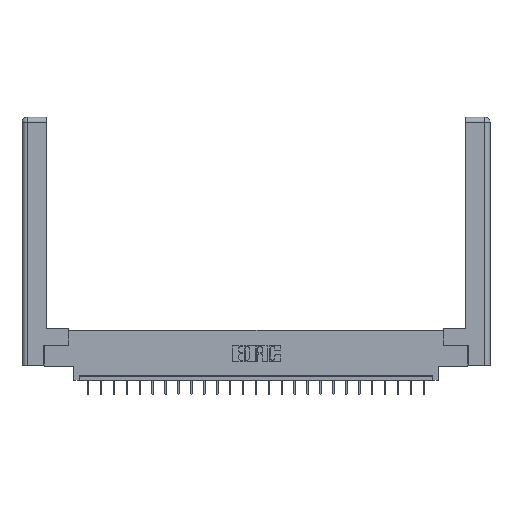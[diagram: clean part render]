
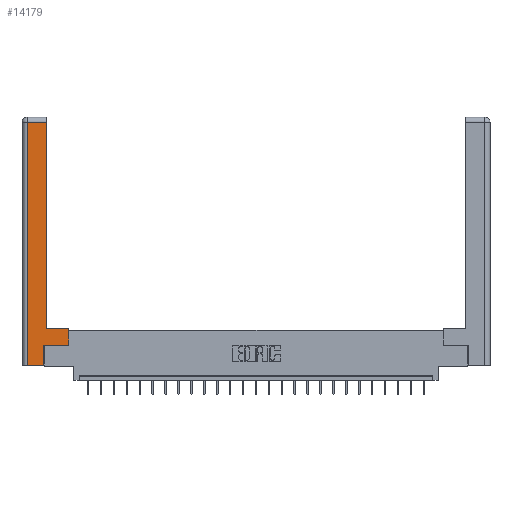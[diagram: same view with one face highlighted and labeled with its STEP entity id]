
A CAD part, top view. The second image highlights one B-rep face of the part: STEP entity #14179.
In plain terms, the highlighted planar face has unit normal (0, 0, 1).
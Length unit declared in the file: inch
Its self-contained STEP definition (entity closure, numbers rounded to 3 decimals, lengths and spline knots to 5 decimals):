
#237 = ORIENTED_EDGE ( 'NONE', *, *, #5616, .T. ) ;
#306 = CARTESIAN_POINT ( 'NONE',  ( 0.265, 0.245, 0. ) ) ;
#751 = VECTOR ( 'NONE', #7410, 39.37008 ) ;
#1029 = VECTOR ( 'NONE', #24122, 39.37008 ) ;
#1068 = VERTEX_POINT ( 'NONE', #18062 ) ;
#2059 = ORIENTED_EDGE ( 'NONE', *, *, #8962, .T. ) ;
#2095 = DIRECTION ( 'NONE',  ( -1., 0., 0. ) ) ;
#2140 = LINE ( 'NONE', #4128, #20501 ) ;
#3215 = FACE_OUTER_BOUND ( 'NONE', #4001, .T. ) ;
#3559 = DIRECTION ( 'NONE',  ( 1., 0., 0. ) ) ;
#3942 = LINE ( 'NONE', #7046, #16914 ) ;
#4001 = EDGE_LOOP ( 'NONE', ( #12333, #2059, #17284, #21267, #6269, #237, #24018, #21779 ) ) ;
#4022 = VECTOR ( 'NONE', #21543, 39.37008 ) ;
#4128 = CARTESIAN_POINT ( 'NONE',  ( 0.0615, 2.94, 0. ) ) ;
#4380 = EDGE_CURVE ( 'NONE', #19378, #19772, #11286, .T. ) ;
#5436 = CARTESIAN_POINT ( 'NONE',  ( 0.565, 0.245, 0. ) ) ;
#5616 = EDGE_CURVE ( 'NONE', #1068, #10010, #20565, .T. ) ;
#5672 = LINE ( 'NONE', #22500, #24684 ) ;
#5932 = DIRECTION ( 'NONE',  ( -1., 0., 0. ) ) ;
#6062 = DIRECTION ( 'NONE',  ( 1., 0., 0. ) ) ;
#6269 = ORIENTED_EDGE ( 'NONE', *, *, #20833, .T. ) ;
#7012 = CARTESIAN_POINT ( 'NONE',  ( 0.565, 0.45, 0. ) ) ;
#7046 = CARTESIAN_POINT ( 'NONE',  ( 0.295, 3., 0. ) ) ;
#7410 = DIRECTION ( 'NONE',  ( 0., -1., 0. ) ) ;
#7493 = CARTESIAN_POINT ( 'NONE',  ( 0.295, 2.94, 0. ) ) ;
#7655 = LINE ( 'NONE', #10740, #1029 ) ;
#8755 = DIRECTION ( 'NONE',  ( -1., 0., 0. ) ) ;
#8962 = EDGE_CURVE ( 'NONE', #15490, #19378, #2140, .T. ) ;
#10010 = VERTEX_POINT ( 'NONE', #13525 ) ;
#10452 = LINE ( 'NONE', #15320, #11635 ) ;
#10674 = VERTEX_POINT ( 'NONE', #21814 ) ;
#10740 = CARTESIAN_POINT ( 'NONE',  ( 0.565, 0.45, 0. ) ) ;
#11286 = LINE ( 'NONE', #19085, #751 ) ;
#11635 = VECTOR ( 'NONE', #6062, 39.37008 ) ;
#11883 = CARTESIAN_POINT ( 'NONE',  ( 0., 0., 0. ) ) ;
#12333 = ORIENTED_EDGE ( 'NONE', *, *, #22067, .T. ) ;
#13169 = EDGE_CURVE ( 'NONE', #22651, #15896, #5672, .T. ) ;
#13525 = CARTESIAN_POINT ( 'NONE',  ( 0.565, 0.245, 0. ) ) ;
#13870 = CARTESIAN_POINT ( 'NONE',  ( 0.0615, 2.94, 0. ) ) ;
#14179 = ADVANCED_FACE ( 'NONE', ( #3215 ), #17454, .F. ) ;
#14296 = EDGE_CURVE ( 'NONE', #19772, #10674, #10452, .T. ) ;
#14885 = AXIS2_PLACEMENT_3D ( 'NONE', #11883, #19299, #5932 ) ;
#15320 = CARTESIAN_POINT ( 'NONE',  ( 0.265, 0., 0. ) ) ;
#15430 = CARTESIAN_POINT ( 'NONE',  ( 0.295, 0.45, 0. ) ) ;
#15489 = LINE ( 'NONE', #306, #4022 ) ;
#15490 = VERTEX_POINT ( 'NONE', #7493 ) ;
#15896 = VERTEX_POINT ( 'NONE', #15430 ) ;
#16914 = VECTOR ( 'NONE', #22372, 39.37008 ) ;
#17284 = ORIENTED_EDGE ( 'NONE', *, *, #4380, .T. ) ;
#17454 = PLANE ( 'NONE',  #14885 ) ;
#18062 = CARTESIAN_POINT ( 'NONE',  ( 0.265, 0.245, 0. ) ) ;
#18195 = VECTOR ( 'NONE', #3559, 39.37008 ) ;
#19085 = CARTESIAN_POINT ( 'NONE',  ( 0.0615, 0., 0. ) ) ;
#19299 = DIRECTION ( 'NONE',  ( 0., 0., -1. ) ) ;
#19378 = VERTEX_POINT ( 'NONE', #13870 ) ;
#19772 = VERTEX_POINT ( 'NONE', #23060 ) ;
#19919 = EDGE_CURVE ( 'NONE', #10010, #22651, #7655, .T. ) ;
#20501 = VECTOR ( 'NONE', #2095, 39.37008 ) ;
#20565 = LINE ( 'NONE', #5436, #18195 ) ;
#20833 = EDGE_CURVE ( 'NONE', #10674, #1068, #15489, .T. ) ;
#21267 = ORIENTED_EDGE ( 'NONE', *, *, #14296, .T. ) ;
#21543 = DIRECTION ( 'NONE',  ( 0., 1., 0. ) ) ;
#21779 = ORIENTED_EDGE ( 'NONE', *, *, #13169, .T. ) ;
#21814 = CARTESIAN_POINT ( 'NONE',  ( 0.265, 0., 0. ) ) ;
#22067 = EDGE_CURVE ( 'NONE', #15896, #15490, #3942, .T. ) ;
#22372 = DIRECTION ( 'NONE',  ( 0., 1., 0. ) ) ;
#22500 = CARTESIAN_POINT ( 'NONE',  ( 0.295, 0.45, 0. ) ) ;
#22651 = VERTEX_POINT ( 'NONE', #7012 ) ;
#23060 = CARTESIAN_POINT ( 'NONE',  ( 0.0615, 0., 0. ) ) ;
#24018 = ORIENTED_EDGE ( 'NONE', *, *, #19919, .T. ) ;
#24122 = DIRECTION ( 'NONE',  ( 0., 1., 0. ) ) ;
#24684 = VECTOR ( 'NONE', #8755, 39.37008 ) ;
